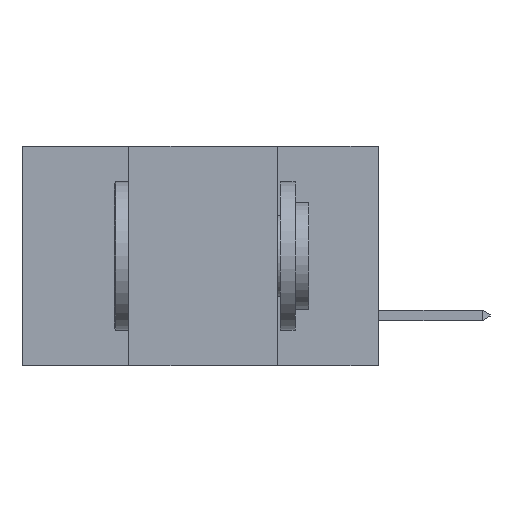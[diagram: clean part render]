
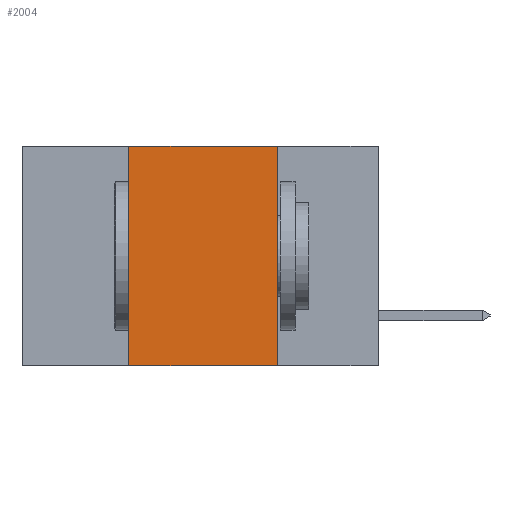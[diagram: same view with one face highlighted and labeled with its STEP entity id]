
A CAD part, left-side view. The second image highlights one B-rep face of the part: STEP entity #2004.
In plain terms, the highlighted planar face has unit normal (-1, 0, 0).
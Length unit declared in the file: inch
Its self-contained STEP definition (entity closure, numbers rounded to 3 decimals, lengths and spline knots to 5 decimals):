
#367 = DIRECTION ( 'NONE',  ( 0., -1., 0. ) ) ;
#1016 = CARTESIAN_POINT ( 'NONE',  ( 0., 0.6, -0.37 ) ) ;
#1544 = CARTESIAN_POINT ( 'NONE',  ( 0., 0.42, -0.37 ) ) ;
#1715 = EDGE_CURVE ( 'NONE', #4589, #15658, #13861, .T. ) ;
#1784 = DIRECTION ( 'NONE',  ( 1., 0., 0. ) ) ;
#2004 = ADVANCED_FACE ( 'NONE', ( #16629 ), #9773, .F. ) ;
#2036 = ORIENTED_EDGE ( 'NONE', *, *, #7040, .F. ) ;
#2096 = VECTOR ( 'NONE', #367, 39.37008 ) ;
#2163 = LINE ( 'NONE', #4438, #8790 ) ;
#2434 = ORIENTED_EDGE ( 'NONE', *, *, #3511, .F. ) ;
#2520 = CARTESIAN_POINT ( 'NONE',  ( 0., 0.42, 0. ) ) ;
#3511 = EDGE_CURVE ( 'NONE', #13436, #4589, #11055, .T. ) ;
#3648 = DIRECTION ( 'NONE',  ( 0., 0., -1. ) ) ;
#4239 = DIRECTION ( 'NONE',  ( 0., 0., 1. ) ) ;
#4438 = CARTESIAN_POINT ( 'NONE',  ( 0., 0.42, -0.37 ) ) ;
#4589 = VERTEX_POINT ( 'NONE', #11204 ) ;
#4946 = CARTESIAN_POINT ( 'NONE',  ( 0., 0.17, -0.37 ) ) ;
#5153 = DIRECTION ( 'NONE',  ( 0., -1., 0. ) ) ;
#5411 = CARTESIAN_POINT ( 'NONE',  ( 0., 0.6, 0. ) ) ;
#5755 = VERTEX_POINT ( 'NONE', #1544 ) ;
#6183 = AXIS2_PLACEMENT_3D ( 'NONE', #15312, #1784, #15836 ) ;
#6822 = ORIENTED_EDGE ( 'NONE', *, *, #1715, .F. ) ;
#7040 = EDGE_CURVE ( 'NONE', #5755, #13436, #2163, .T. ) ;
#7537 = VECTOR ( 'NONE', #5153, 39.37008 ) ;
#8790 = VECTOR ( 'NONE', #4239, 39.37008 ) ;
#8808 = EDGE_CURVE ( 'NONE', #5755, #15658, #9584, .T. ) ;
#9584 = LINE ( 'NONE', #1016, #2096 ) ;
#9773 = PLANE ( 'NONE',  #6183 ) ;
#9958 = CARTESIAN_POINT ( 'NONE',  ( 0., 0.17, -0.37 ) ) ;
#10495 = VECTOR ( 'NONE', #3648, 39.37008 ) ;
#11055 = LINE ( 'NONE', #5411, #7537 ) ;
#11204 = CARTESIAN_POINT ( 'NONE',  ( 0., 0.17, 0. ) ) ;
#11894 = EDGE_LOOP ( 'NONE', ( #6822, #2434, #2036, #12734 ) ) ;
#12734 = ORIENTED_EDGE ( 'NONE', *, *, #8808, .T. ) ;
#13436 = VERTEX_POINT ( 'NONE', #2520 ) ;
#13861 = LINE ( 'NONE', #4946, #10495 ) ;
#15312 = CARTESIAN_POINT ( 'NONE',  ( 0., 0.6, 0. ) ) ;
#15658 = VERTEX_POINT ( 'NONE', #9958 ) ;
#15836 = DIRECTION ( 'NONE',  ( 0., 0., -1. ) ) ;
#16629 = FACE_OUTER_BOUND ( 'NONE', #11894, .T. ) ;
